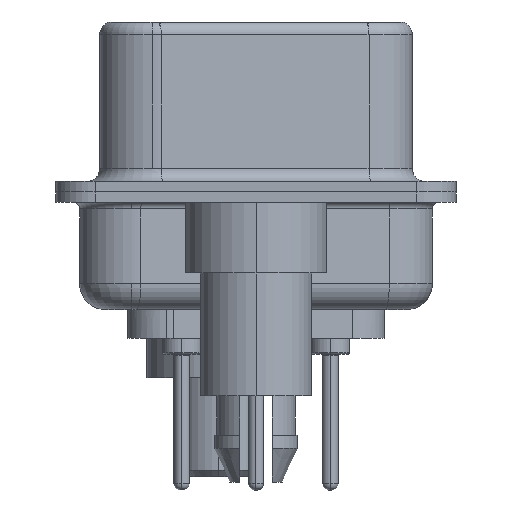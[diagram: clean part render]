
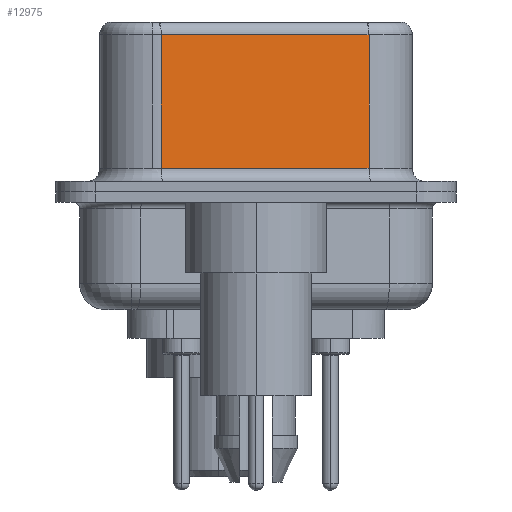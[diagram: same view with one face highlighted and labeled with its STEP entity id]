
A CAD part, left-side view. The second image highlights one B-rep face of the part: STEP entity #12975.
In plain terms, the highlighted planar face has unit normal (-0.985, -0.174, 0).
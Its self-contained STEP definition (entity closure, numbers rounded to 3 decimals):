
#1093 = EDGE_CURVE ( 'NONE', #19680, #22377, #2978, .T. ) ;
#2291 = DIRECTION ( 'NONE',  ( 0.985, 0.174, 0. ) ) ;
#2978 = LINE ( 'NONE', #27819, #23548 ) ;
#3537 = VECTOR ( 'NONE', #27050, 1000. ) ;
#3567 = CARTESIAN_POINT ( 'NONE',  ( 5.132, -4.322, 0.9 ) ) ;
#3598 = EDGE_CURVE ( 'NONE', #10960, #22377, #14585, .T. ) ;
#4244 = DIRECTION ( 'NONE',  ( 0., 0., -1. ) ) ;
#4572 = DIRECTION ( 'NONE',  ( -0.174, 0.985, 0. ) ) ;
#5338 = LINE ( 'NONE', #25984, #25887 ) ;
#6083 = FACE_OUTER_BOUND ( 'NONE', #28266, .T. ) ;
#6624 = CARTESIAN_POINT ( 'NONE',  ( 5.132, -4.322, 6.52 ) ) ;
#8744 = CARTESIAN_POINT ( 'NONE',  ( 3.73, 3.628, 0.9 ) ) ;
#9569 = ORIENTED_EDGE ( 'NONE', *, *, #15513, .T. ) ;
#10960 = VERTEX_POINT ( 'NONE', #8744 ) ;
#12534 = VERTEX_POINT ( 'NONE', #14713 ) ;
#12975 = ADVANCED_FACE ( 'NONE', ( #6083 ), #13842, .F. ) ;
#13093 = CARTESIAN_POINT ( 'NONE',  ( 5.132, -4.322, 0.9 ) ) ;
#13842 = PLANE ( 'NONE',  #28874 ) ;
#14197 = ORIENTED_EDGE ( 'NONE', *, *, #3598, .T. ) ;
#14333 = DIRECTION ( 'NONE',  ( 0., 0., -1. ) ) ;
#14585 = LINE ( 'NONE', #3567, #3537 ) ;
#14713 = CARTESIAN_POINT ( 'NONE',  ( 3.73, 3.628, 6.02 ) ) ;
#15513 = EDGE_CURVE ( 'NONE', #12534, #10960, #5338, .T. ) ;
#15876 = CARTESIAN_POINT ( 'NONE',  ( 5.132, -4.322, 6.02 ) ) ;
#16893 = EDGE_CURVE ( 'NONE', #19680, #12534, #26217, .T. ) ;
#19058 = DIRECTION ( 'NONE',  ( -0.174, 0.985, 0. ) ) ;
#19680 = VERTEX_POINT ( 'NONE', #15876 ) ;
#21342 = ORIENTED_EDGE ( 'NONE', *, *, #1093, .F. ) ;
#22377 = VERTEX_POINT ( 'NONE', #13093 ) ;
#23548 = VECTOR ( 'NONE', #4244, 1000. ) ;
#24184 = ORIENTED_EDGE ( 'NONE', *, *, #16893, .T. ) ;
#25483 = VECTOR ( 'NONE', #19058, 1000. ) ;
#25588 = CARTESIAN_POINT ( 'NONE',  ( 5.132, -4.322, 6.02 ) ) ;
#25887 = VECTOR ( 'NONE', #14333, 1000. ) ;
#25984 = CARTESIAN_POINT ( 'NONE',  ( 3.73, 3.628, 6.52 ) ) ;
#26217 = LINE ( 'NONE', #25588, #25483 ) ;
#27050 = DIRECTION ( 'NONE',  ( 0.174, -0.985, 0. ) ) ;
#27819 = CARTESIAN_POINT ( 'NONE',  ( 5.132, -4.322, 6.52 ) ) ;
#28266 = EDGE_LOOP ( 'NONE', ( #21342, #24184, #9569, #14197 ) ) ;
#28874 = AXIS2_PLACEMENT_3D ( 'NONE', #6624, #2291, #4572 ) ;
